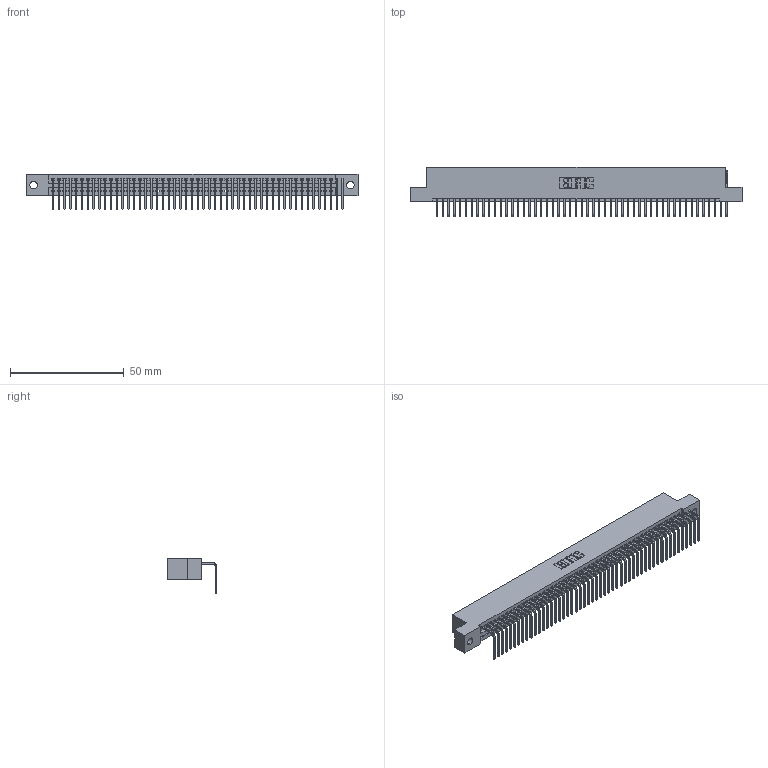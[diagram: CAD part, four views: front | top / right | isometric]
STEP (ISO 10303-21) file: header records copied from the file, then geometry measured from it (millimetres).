
FILE_DESCRIPTION (( 'STEP AP203' ), '1' );
FILE_NAME ('345-051-558-102.STEP', '2019-10-10T18:28:44', ( '' ), ( '' ), 'SwSTEP 2.0', 'SolidWorks 2016', '' );
FILE_SCHEMA (( 'CONFIG_CONTROL_DESIGN' ));
Length unit declared in the file: inch
Products named in the file (3): 345 Part_Flush Mounting Lugs - 0.128 Dia; 345-292-001_558 Tail - 2; 345-051-558-102
Assembly tree (52 placements, depth 2):
  345-051-558-102
    345 Part_Flush Mounting Lugs - 0.128 Dia
    345-292-001_558 Tail - 2  x51
Bounding box: 145.67 x 21.83 x 15.37 mm (x, y, z)
Volume: 14049.3 mm3; surface area: 19613.9 mm2
Topology: 52 solids, 52 shells, 3154 faces, 9515 edges, 6274 vertices
Faces by surface type: plane 2194, cylinder 960
Entity records: 36087 total; most frequent: CARTESIAN_POINT 6249, ORIENTED_EDGE 6230, DIRECTION 5449, EDGE_CURVE 3115, LINE 2787, VECTOR 2787, VERTEX_POINT 2074, AXIS2_PLACEMENT_3D 1331
